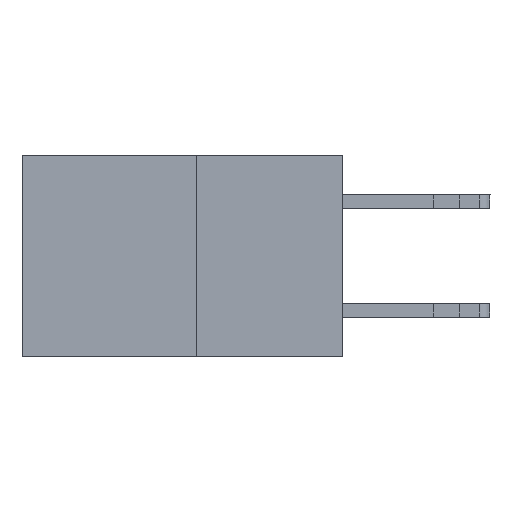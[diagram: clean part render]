
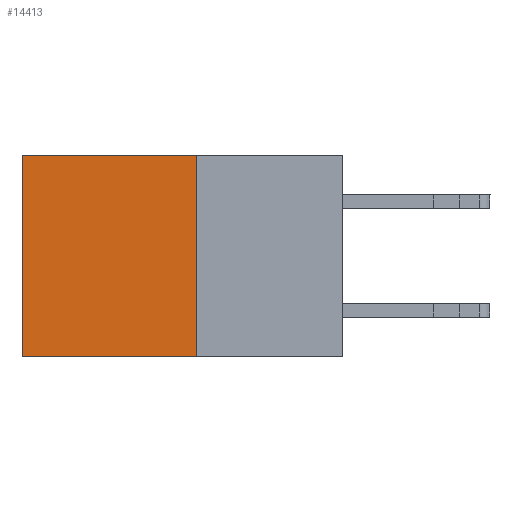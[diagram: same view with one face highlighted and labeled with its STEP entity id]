
A CAD part, left-side view. The second image highlights one B-rep face of the part: STEP entity #14413.
In plain terms, the highlighted planar face has unit normal (-1, 0, 0).
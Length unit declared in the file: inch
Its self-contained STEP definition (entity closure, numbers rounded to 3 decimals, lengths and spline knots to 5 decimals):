
#537 = EDGE_CURVE ( 'NONE', #13409, #12758, #12338, .T. ) ;
#3012 = PLANE ( 'NONE',  #24542 ) ;
#3088 = CARTESIAN_POINT ( 'NONE',  ( 0.277, 0.27, 0. ) ) ;
#4491 = VERTEX_POINT ( 'NONE', #15428 ) ;
#4903 = VECTOR ( 'NONE', #5582, 39.37008 ) ;
#5024 = CARTESIAN_POINT ( 'NONE',  ( 0.277, 0.59, 0. ) ) ;
#5491 = CARTESIAN_POINT ( 'NONE',  ( 0.277, 0.27, -0.37 ) ) ;
#5582 = DIRECTION ( 'NONE',  ( 0., 1., 0. ) ) ;
#5709 = EDGE_CURVE ( 'NONE', #18509, #4491, #10660, .T. ) ;
#5722 = DIRECTION ( 'NONE',  ( 0., 0., -1. ) ) ;
#7703 = LINE ( 'NONE', #5491, #14239 ) ;
#7985 = ORIENTED_EDGE ( 'NONE', *, *, #24362, .T. ) ;
#9483 = DIRECTION ( 'NONE',  ( 1., 0., 0. ) ) ;
#10660 = LINE ( 'NONE', #28632, #11048 ) ;
#11048 = VECTOR ( 'NONE', #26025, 39.37008 ) ;
#11106 = VECTOR ( 'NONE', #5722, 39.37008 ) ;
#11921 = LINE ( 'NONE', #3088, #4903 ) ;
#11972 = DIRECTION ( 'NONE',  ( 0., 0., -1. ) ) ;
#12338 = LINE ( 'NONE', #23974, #11106 ) ;
#12758 = VERTEX_POINT ( 'NONE', #19401 ) ;
#13409 = VERTEX_POINT ( 'NONE', #5024 ) ;
#13598 = CARTESIAN_POINT ( 'NONE',  ( 0.277, 0.27, -0.37 ) ) ;
#13893 = ORIENTED_EDGE ( 'NONE', *, *, #15247, .F. ) ;
#14239 = VECTOR ( 'NONE', #27738, 39.37008 ) ;
#14413 = ADVANCED_FACE ( 'NONE', ( #23194 ), #3012, .F. ) ;
#15247 = EDGE_CURVE ( 'NONE', #4491, #12758, #7703, .T. ) ;
#15428 = CARTESIAN_POINT ( 'NONE',  ( 0.277, 0.27, -0.37 ) ) ;
#18509 = VERTEX_POINT ( 'NONE', #22710 ) ;
#19401 = CARTESIAN_POINT ( 'NONE',  ( 0.277, 0.59, -0.37 ) ) ;
#22710 = CARTESIAN_POINT ( 'NONE',  ( 0.277, 0.27, 0. ) ) ;
#23194 = FACE_OUTER_BOUND ( 'NONE', #25385, .T. ) ;
#23974 = CARTESIAN_POINT ( 'NONE',  ( 0.277, 0.59, -0.37 ) ) ;
#24362 = EDGE_CURVE ( 'NONE', #18509, #13409, #11921, .T. ) ;
#24542 = AXIS2_PLACEMENT_3D ( 'NONE', #13598, #9483, #11972 ) ;
#25385 = EDGE_LOOP ( 'NONE', ( #28278, #13893, #26462, #7985 ) ) ;
#26025 = DIRECTION ( 'NONE',  ( 0., 0., -1. ) ) ;
#26462 = ORIENTED_EDGE ( 'NONE', *, *, #5709, .F. ) ;
#27738 = DIRECTION ( 'NONE',  ( 0., 1., 0. ) ) ;
#28278 = ORIENTED_EDGE ( 'NONE', *, *, #537, .T. ) ;
#28632 = CARTESIAN_POINT ( 'NONE',  ( 0.277, 0.27, -0.37 ) ) ;
